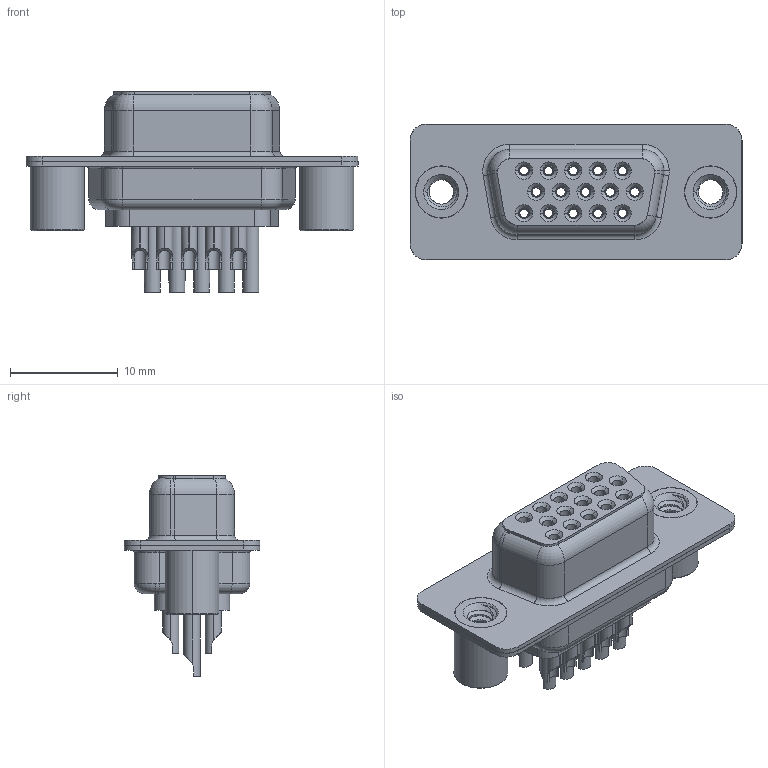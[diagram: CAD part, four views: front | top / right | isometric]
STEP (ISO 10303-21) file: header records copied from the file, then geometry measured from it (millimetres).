
FILE_DESCRIPTION (( 'STEP AP203' ), '1' );
FILE_NAME ('638-015-632-249.STEP', '2020-07-18T19:24:44', ( '' ), ( '' ), 'SwSTEP 2.0', 'SolidWorks 2020', '' );
FILE_SCHEMA (( 'CONFIG_CONTROL_DESIGN' ));
Length unit declared in the file: millimetre
Products named in the file (8): 638 Contact Row 3_32; 638 Contact Row 1_32; 638 Contact Row 2_32; 638-015-632-249; 638 Shell Front_15 Contacts; 638 Housing_15 Contacts; 638 Shell Rear_15 Contacts; 638 4-40 Threaded Standoff BS
Assembly tree (20 placements, depth 2):
  638-015-632-249
    638 Housing_15 Contacts
    638 Shell Front_15 Contacts
    638 Shell Rear_15 Contacts
    638 Contact Row 1_32  x5
    638 Contact Row 2_32  x5
    638 Contact Row 3_32  x5
    638 4-40 Threaded Standoff BS  x2
Bounding box: 30.81 x 12.6 x 18.6 mm (x, y, z)
Volume: 1698.9 mm3; surface area: 6049.7 mm2
Topology: 20 solids, 20 shells, 1636 faces, 4139 edges, 2599 vertices
Faces by surface type: cylinder 532, plane 382, torus 327, bspline 306, cone 89
Entity records: 25122 total; most frequent: CARTESIAN_POINT 8169, DIRECTION 3350, ORIENTED_EDGE 3300, EDGE_CURVE 1650, AXIS2_PLACEMENT_3D 1388, VERTEX_POINT 1038, EDGE_LOOP 778, CIRCLE 748
